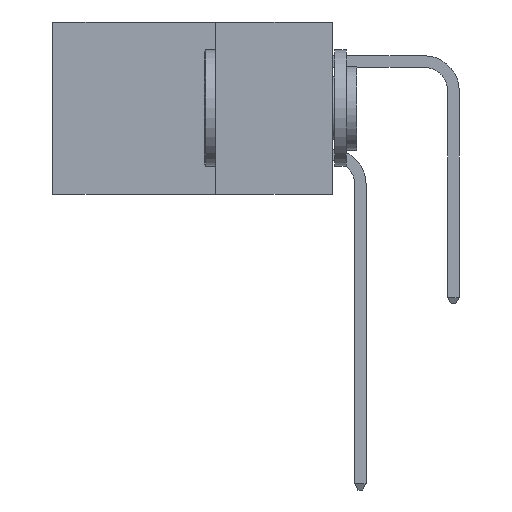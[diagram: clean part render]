
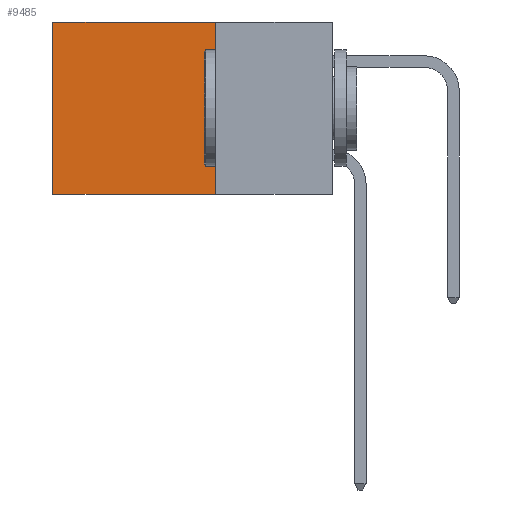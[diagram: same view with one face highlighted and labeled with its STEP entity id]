
A CAD part, left-side view. The second image highlights one B-rep face of the part: STEP entity #9485.
In plain terms, the highlighted planar face has unit normal (-1, 0, 0).
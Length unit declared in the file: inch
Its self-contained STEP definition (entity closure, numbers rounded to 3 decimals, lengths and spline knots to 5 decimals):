
#386 = EDGE_CURVE ( 'NONE', #6692, #4918, #947, .T. ) ;
#552 = VECTOR ( 'NONE', #14325, 39.37008 ) ;
#947 = LINE ( 'NONE', #12199, #13128 ) ;
#2268 = CARTESIAN_POINT ( 'NONE',  ( 0.2615, 0.6, 0. ) ) ;
#3169 = EDGE_CURVE ( 'NONE', #14575, #4918, #7023, .T. ) ;
#4275 = CARTESIAN_POINT ( 'NONE',  ( 0.2615, 0.6, -0.37 ) ) ;
#4566 = EDGE_LOOP ( 'NONE', ( #6095, #6158, #6202, #6273 ) ) ;
#4918 = VERTEX_POINT ( 'NONE', #4275 ) ;
#5067 = DIRECTION ( 'NONE',  ( 0., 1., 0. ) ) ;
#5219 = PLANE ( 'NONE',  #6266 ) ;
#5268 = DIRECTION ( 'NONE',  ( 1., 0., 0. ) ) ;
#6095 = ORIENTED_EDGE ( 'NONE', *, *, #3169, .T. ) ;
#6158 = ORIENTED_EDGE ( 'NONE', *, *, #386, .F. ) ;
#6202 = ORIENTED_EDGE ( 'NONE', *, *, #14089, .F. ) ;
#6266 = AXIS2_PLACEMENT_3D ( 'NONE', #12366, #5268, #13488 ) ;
#6273 = ORIENTED_EDGE ( 'NONE', *, *, #12409, .T. ) ;
#6692 = VERTEX_POINT ( 'NONE', #8043 ) ;
#7023 = LINE ( 'NONE', #10659, #13211 ) ;
#7477 = CARTESIAN_POINT ( 'NONE',  ( 0.2615, 0.25, -0.37 ) ) ;
#8043 = CARTESIAN_POINT ( 'NONE',  ( 0.2615, 0.25, -0.37 ) ) ;
#8484 = VECTOR ( 'NONE', #5067, 39.37008 ) ;
#9132 = CARTESIAN_POINT ( 'NONE',  ( 0.2615, 0.25, 0. ) ) ;
#9485 = ADVANCED_FACE ( 'NONE', ( #10919 ), #5219, .F. ) ;
#10244 = VERTEX_POINT ( 'NONE', #9132 ) ;
#10659 = CARTESIAN_POINT ( 'NONE',  ( 0.2615, 0.6, -0.37 ) ) ;
#10919 = FACE_OUTER_BOUND ( 'NONE', #4566, .T. ) ;
#11672 = DIRECTION ( 'NONE',  ( 0., 0., -1. ) ) ;
#12199 = CARTESIAN_POINT ( 'NONE',  ( 0.2615, 0.25, -0.37 ) ) ;
#12366 = CARTESIAN_POINT ( 'NONE',  ( 0.2615, 0.25, -0.37 ) ) ;
#12409 = EDGE_CURVE ( 'NONE', #10244, #14575, #14174, .T. ) ;
#12676 = DIRECTION ( 'NONE',  ( 0., 1., 0. ) ) ;
#13109 = LINE ( 'NONE', #7477, #552 ) ;
#13128 = VECTOR ( 'NONE', #12676, 39.37008 ) ;
#13211 = VECTOR ( 'NONE', #11672, 39.37008 ) ;
#13318 = CARTESIAN_POINT ( 'NONE',  ( 0.2615, 0.25, 0. ) ) ;
#13488 = DIRECTION ( 'NONE',  ( 0., 0., -1. ) ) ;
#14089 = EDGE_CURVE ( 'NONE', #10244, #6692, #13109, .T. ) ;
#14174 = LINE ( 'NONE', #13318, #8484 ) ;
#14325 = DIRECTION ( 'NONE',  ( 0., 0., -1. ) ) ;
#14575 = VERTEX_POINT ( 'NONE', #2268 ) ;
